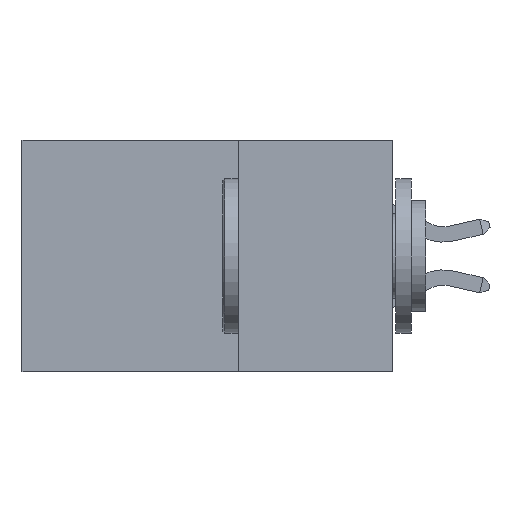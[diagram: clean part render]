
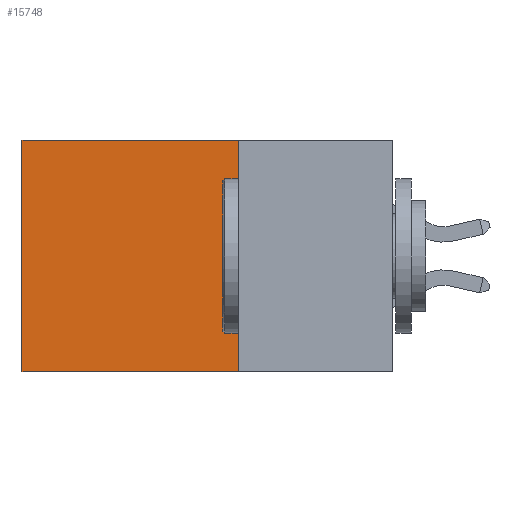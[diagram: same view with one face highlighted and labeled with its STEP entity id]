
A CAD part, left-side view. The second image highlights one B-rep face of the part: STEP entity #15748.
In plain terms, the highlighted planar face has unit normal (-1, 0, 0).
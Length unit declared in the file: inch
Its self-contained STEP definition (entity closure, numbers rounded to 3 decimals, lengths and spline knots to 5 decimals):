
#292 = LINE ( 'NONE', #4077, #15995 ) ;
#929 = AXIS2_PLACEMENT_3D ( 'NONE', #12809, #2142, #9846 ) ;
#1122 = VECTOR ( 'NONE', #1716, 39.37008 ) ;
#1592 = LINE ( 'NONE', #9268, #1122 ) ;
#1716 = DIRECTION ( 'NONE',  ( 0., 1., 0. ) ) ;
#2142 = DIRECTION ( 'NONE',  ( 1., 0., 0. ) ) ;
#2958 = DIRECTION ( 'NONE',  ( 0., 1., 0. ) ) ;
#4024 = CARTESIAN_POINT ( 'NONE',  ( 0.2875, 0.6, -0.375 ) ) ;
#4077 = CARTESIAN_POINT ( 'NONE',  ( 0.2875, 0.6, -0.375 ) ) ;
#6420 = EDGE_CURVE ( 'NONE', #6594, #7884, #1592, .T. ) ;
#6593 = CARTESIAN_POINT ( 'NONE',  ( 0.2875, 0.25, -0.375 ) ) ;
#6594 = VERTEX_POINT ( 'NONE', #8186 ) ;
#6787 = VERTEX_POINT ( 'NONE', #4024 ) ;
#7469 = LINE ( 'NONE', #18554, #17936 ) ;
#7884 = VERTEX_POINT ( 'NONE', #14132 ) ;
#8147 = EDGE_CURVE ( 'NONE', #10474, #6787, #18934, .T. ) ;
#8186 = CARTESIAN_POINT ( 'NONE',  ( 0.2875, 0.25, 0. ) ) ;
#9268 = CARTESIAN_POINT ( 'NONE',  ( 0.2875, 0.25, 0. ) ) ;
#9846 = DIRECTION ( 'NONE',  ( 0., 0., -1. ) ) ;
#9910 = VECTOR ( 'NONE', #2958, 39.37008 ) ;
#10172 = DIRECTION ( 'NONE',  ( 0., 0., -1. ) ) ;
#10474 = VERTEX_POINT ( 'NONE', #6593 ) ;
#10506 = EDGE_LOOP ( 'NONE', ( #19238, #10890, #16231, #16154 ) ) ;
#10890 = ORIENTED_EDGE ( 'NONE', *, *, #8147, .F. ) ;
#12809 = CARTESIAN_POINT ( 'NONE',  ( 0.2875, 0.25, -0.375 ) ) ;
#13282 = EDGE_CURVE ( 'NONE', #7884, #6787, #292, .T. ) ;
#14128 = DIRECTION ( 'NONE',  ( 0., 0., -1. ) ) ;
#14132 = CARTESIAN_POINT ( 'NONE',  ( 0.2875, 0.6, 0. ) ) ;
#14317 = PLANE ( 'NONE',  #929 ) ;
#15748 = ADVANCED_FACE ( 'NONE', ( #16275 ), #14317, .F. ) ;
#15995 = VECTOR ( 'NONE', #10172, 39.37008 ) ;
#16154 = ORIENTED_EDGE ( 'NONE', *, *, #6420, .T. ) ;
#16231 = ORIENTED_EDGE ( 'NONE', *, *, #16647, .F. ) ;
#16275 = FACE_OUTER_BOUND ( 'NONE', #10506, .T. ) ;
#16647 = EDGE_CURVE ( 'NONE', #6594, #10474, #7469, .T. ) ;
#16711 = CARTESIAN_POINT ( 'NONE',  ( 0.2875, 0.25, -0.375 ) ) ;
#17936 = VECTOR ( 'NONE', #14128, 39.37008 ) ;
#18554 = CARTESIAN_POINT ( 'NONE',  ( 0.2875, 0.25, -0.375 ) ) ;
#18934 = LINE ( 'NONE', #16711, #9910 ) ;
#19238 = ORIENTED_EDGE ( 'NONE', *, *, #13282, .T. ) ;
